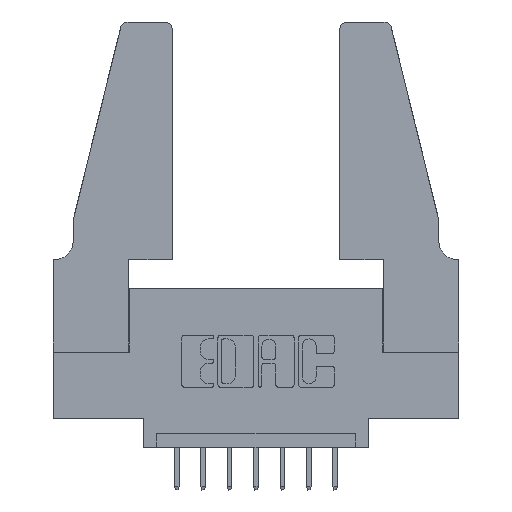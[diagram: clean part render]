
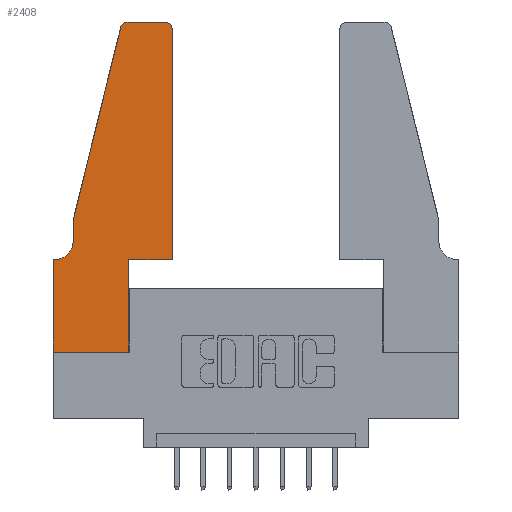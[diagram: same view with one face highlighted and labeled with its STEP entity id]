
A CAD part, top view. The second image highlights one B-rep face of the part: STEP entity #2408.
In plain terms, the highlighted planar face has unit normal (0, 0, 1).
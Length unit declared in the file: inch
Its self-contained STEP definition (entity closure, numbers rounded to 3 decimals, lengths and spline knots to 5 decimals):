
#80 = VECTOR ( 'NONE', #2975, 39.37008 ) ;
#292 = EDGE_CURVE ( 'NONE', #4403, #4532, #450, .T. ) ;
#304 = ORIENTED_EDGE ( 'NONE', *, *, #3924, .T. ) ;
#388 = CARTESIAN_POINT ( 'NONE',  ( 0.284, 1.25, 0.37 ) ) ;
#435 = CIRCLE ( 'NONE', #6456, 0.07 ) ;
#450 = LINE ( 'NONE', #4859, #4767 ) ;
#508 = VERTEX_POINT ( 'NONE', #8807 ) ;
#672 = EDGE_CURVE ( 'NONE', #9773, #4466, #435, .T. ) ;
#706 = CARTESIAN_POINT ( 'NONE',  ( 0.0755, 0.35, 0.37 ) ) ;
#926 = CARTESIAN_POINT ( 'NONE',  ( 0.0755, 0.5, 0.37 ) ) ;
#940 = DIRECTION ( 'NONE',  ( 1., 0., 0. ) ) ;
#1115 = CIRCLE ( 'NONE', #2092, 0.03 ) ;
#1356 = DIRECTION ( 'NONE',  ( -1., 0., 0. ) ) ;
#1424 = DIRECTION ( 'NONE',  ( 1., 0., 0. ) ) ;
#1715 = ORIENTED_EDGE ( 'NONE', *, *, #3723, .T. ) ;
#1742 = CARTESIAN_POINT ( 'NONE',  ( 0., 0.35, 0.37 ) ) ;
#1749 = CARTESIAN_POINT ( 'NONE',  ( 0., 0., 0.37 ) ) ;
#1937 = DIRECTION ( 'NONE',  ( 0., -1., 0. ) ) ;
#2003 = CARTESIAN_POINT ( 'NONE',  ( 0.4505, 1.22, 0.37 ) ) ;
#2014 = CARTESIAN_POINT ( 'NONE',  ( 0.2865, 0.35, 0.37 ) ) ;
#2029 = VECTOR ( 'NONE', #8225, 39.37008 ) ;
#2049 = ORIENTED_EDGE ( 'NONE', *, *, #672, .T. ) ;
#2092 = AXIS2_PLACEMENT_3D ( 'NONE', #2285, #11809, #6082 ) ;
#2097 = CARTESIAN_POINT ( 'NONE',  ( 0.0755, 0.5, 0.37 ) ) ;
#2285 = CARTESIAN_POINT ( 'NONE',  ( 0.4205, 1.22, 0.37 ) ) ;
#2408 = ADVANCED_FACE ( 'NONE', ( #4717 ), #11219, .T. ) ;
#2438 = LINE ( 'NONE', #1749, #9279 ) ;
#2567 = EDGE_CURVE ( 'NONE', #8707, #508, #11713, .T. ) ;
#2614 = DIRECTION ( 'NONE',  ( 1., 0., 0. ) ) ;
#2702 = DIRECTION ( 'NONE',  ( 0., 0., 1. ) ) ;
#2924 = EDGE_CURVE ( 'NONE', #7886, #3620, #5779, .T. ) ;
#2963 = CIRCLE ( 'NONE', #3804, 0.03 ) ;
#2975 = DIRECTION ( 'NONE',  ( 0., 1., 0. ) ) ;
#3218 = CARTESIAN_POINT ( 'NONE',  ( 0.0755, 0.42, 0.37 ) ) ;
#3404 = VERTEX_POINT ( 'NONE', #2003 ) ;
#3507 = VECTOR ( 'NONE', #5715, 39.37008 ) ;
#3620 = VERTEX_POINT ( 'NONE', #6560 ) ;
#3641 = LINE ( 'NONE', #9435, #3507 ) ;
#3723 = EDGE_CURVE ( 'NONE', #4466, #8707, #4572, .T. ) ;
#3764 = CARTESIAN_POINT ( 'NONE',  ( 0.4505, 0.35, 0.37 ) ) ;
#3804 = AXIS2_PLACEMENT_3D ( 'NONE', #9997, #7181, #1424 ) ;
#3924 = EDGE_CURVE ( 'NONE', #5905, #9773, #3641, .T. ) ;
#3935 = DIRECTION ( 'NONE',  ( -1., 0., 0. ) ) ;
#4403 = VERTEX_POINT ( 'NONE', #7056 ) ;
#4466 = VERTEX_POINT ( 'NONE', #7975 ) ;
#4532 = VERTEX_POINT ( 'NONE', #388 ) ;
#4572 = LINE ( 'NONE', #706, #2029 ) ;
#4630 = DIRECTION ( 'NONE',  ( 1., 0., 0. ) ) ;
#4717 = FACE_OUTER_BOUND ( 'NONE', #4885, .T. ) ;
#4767 = VECTOR ( 'NONE', #3935, 39.37008 ) ;
#4859 = CARTESIAN_POINT ( 'NONE',  ( 0.2605, 1.25, 0.37 ) ) ;
#4885 = EDGE_LOOP ( 'NONE', ( #12184, #12214, #7704, #304, #2049, #1715, #5255, #8825, #7656, #9828, #10704, #11252 ) ) ;
#5178 = EDGE_CURVE ( 'NONE', #508, #7886, #2438, .T. ) ;
#5255 = ORIENTED_EDGE ( 'NONE', *, *, #2567, .T. ) ;
#5416 = VECTOR ( 'NONE', #6330, 39.37008 ) ;
#5472 = CARTESIAN_POINT ( 'NONE',  ( 0.4505, 0.35, 0.37 ) ) ;
#5539 = EDGE_CURVE ( 'NONE', #7122, #5905, #11056, .T. ) ;
#5685 = VERTEX_POINT ( 'NONE', #10145 ) ;
#5715 = DIRECTION ( 'NONE',  ( 0., -1., 0. ) ) ;
#5739 = CARTESIAN_POINT ( 'NONE',  ( 0., 0., 0.37 ) ) ;
#5779 = LINE ( 'NONE', #2014, #80 ) ;
#5905 = VERTEX_POINT ( 'NONE', #2097 ) ;
#6033 = DIRECTION ( 'NONE',  ( 0., 0., -1. ) ) ;
#6082 = DIRECTION ( 'NONE',  ( 1., 0., 0. ) ) ;
#6330 = DIRECTION ( 'NONE',  ( 0., 1., 0. ) ) ;
#6456 = AXIS2_PLACEMENT_3D ( 'NONE', #11716, #6033, #1356 ) ;
#6560 = CARTESIAN_POINT ( 'NONE',  ( 0.2865, 0.35, 0.37 ) ) ;
#6627 = DIRECTION ( 'NONE',  ( -0.239, -0.971, 0. ) ) ;
#7056 = CARTESIAN_POINT ( 'NONE',  ( 0.4205, 1.25, 0.37 ) ) ;
#7122 = VERTEX_POINT ( 'NONE', #9996 ) ;
#7181 = DIRECTION ( 'NONE',  ( 0., 0., 1. ) ) ;
#7625 = EDGE_CURVE ( 'NONE', #4532, #7122, #2963, .T. ) ;
#7638 = VECTOR ( 'NONE', #6627, 39.37008 ) ;
#7656 = ORIENTED_EDGE ( 'NONE', *, *, #2924, .T. ) ;
#7704 = ORIENTED_EDGE ( 'NONE', *, *, #5539, .T. ) ;
#7886 = VERTEX_POINT ( 'NONE', #11663 ) ;
#7975 = CARTESIAN_POINT ( 'NONE',  ( 0.0055, 0.35, 0.37 ) ) ;
#8225 = DIRECTION ( 'NONE',  ( -1., 0., 0. ) ) ;
#8292 = VECTOR ( 'NONE', #1937, 39.37008 ) ;
#8319 = CARTESIAN_POINT ( 'NONE',  ( 0., 0.35, 0.37 ) ) ;
#8707 = VERTEX_POINT ( 'NONE', #1742 ) ;
#8807 = CARTESIAN_POINT ( 'NONE',  ( 0., 0., 0.37 ) ) ;
#8825 = ORIENTED_EDGE ( 'NONE', *, *, #5178, .T. ) ;
#8912 = EDGE_CURVE ( 'NONE', #3620, #5685, #9635, .T. ) ;
#9279 = VECTOR ( 'NONE', #4630, 39.37008 ) ;
#9435 = CARTESIAN_POINT ( 'NONE',  ( 0.0755, 0.5, 0.37 ) ) ;
#9635 = LINE ( 'NONE', #3764, #10667 ) ;
#9773 = VERTEX_POINT ( 'NONE', #3218 ) ;
#9828 = ORIENTED_EDGE ( 'NONE', *, *, #8912, .T. ) ;
#9996 = CARTESIAN_POINT ( 'NONE',  ( 0.25487, 1.22718, 0.37 ) ) ;
#9997 = CARTESIAN_POINT ( 'NONE',  ( 0.284, 1.22, 0.37 ) ) ;
#10107 = AXIS2_PLACEMENT_3D ( 'NONE', #8319, #2702, #2614 ) ;
#10145 = CARTESIAN_POINT ( 'NONE',  ( 0.4505, 0.35, 0.37 ) ) ;
#10160 = EDGE_CURVE ( 'NONE', #3404, #4403, #1115, .T. ) ;
#10667 = VECTOR ( 'NONE', #940, 39.37008 ) ;
#10704 = ORIENTED_EDGE ( 'NONE', *, *, #11199, .T. ) ;
#10921 = LINE ( 'NONE', #5472, #5416 ) ;
#11056 = LINE ( 'NONE', #926, #7638 ) ;
#11199 = EDGE_CURVE ( 'NONE', #5685, #3404, #10921, .T. ) ;
#11219 = PLANE ( 'NONE',  #10107 ) ;
#11252 = ORIENTED_EDGE ( 'NONE', *, *, #10160, .T. ) ;
#11663 = CARTESIAN_POINT ( 'NONE',  ( 0.2865, 0., 0.37 ) ) ;
#11713 = LINE ( 'NONE', #5739, #8292 ) ;
#11716 = CARTESIAN_POINT ( 'NONE',  ( 0.0055, 0.42, 0.37 ) ) ;
#11809 = DIRECTION ( 'NONE',  ( 0., 0., 1. ) ) ;
#12184 = ORIENTED_EDGE ( 'NONE', *, *, #292, .T. ) ;
#12214 = ORIENTED_EDGE ( 'NONE', *, *, #7625, .T. ) ;
